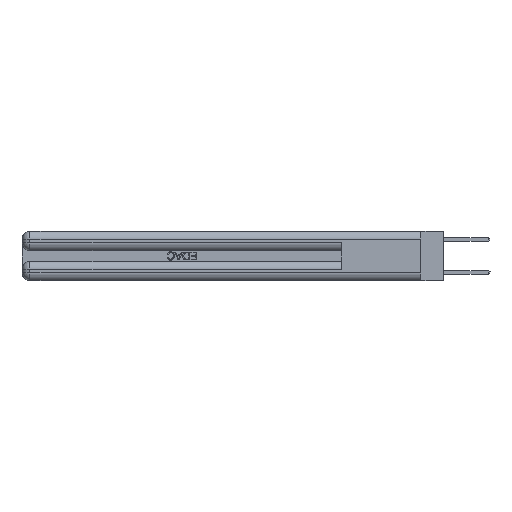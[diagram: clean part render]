
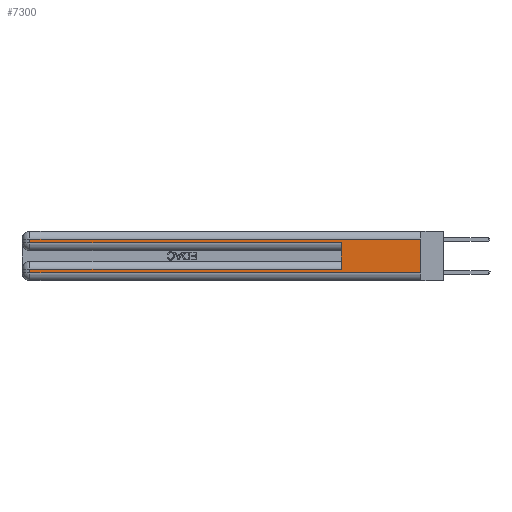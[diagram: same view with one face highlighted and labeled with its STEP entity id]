
A CAD part, left-side view. The second image highlights one B-rep face of the part: STEP entity #7300.
In plain terms, the highlighted planar face has unit normal (-1, 0, 0).
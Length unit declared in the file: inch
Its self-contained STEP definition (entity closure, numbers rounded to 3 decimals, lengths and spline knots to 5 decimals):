
#155 = CARTESIAN_POINT ( 'NONE',  ( 0., 2.94, 0.085 ) ) ;
#1651 = LINE ( 'NONE', #11303, #3616 ) ;
#1743 = CARTESIAN_POINT ( 'NONE',  ( 0., 0.6, 0.085 ) ) ;
#1828 = DIRECTION ( 'NONE',  ( 0., -1., 0. ) ) ;
#3302 = DIRECTION ( 'NONE',  ( 0., 0., -1. ) ) ;
#3616 = VECTOR ( 'NONE', #23784, 39.37008 ) ;
#3754 = EDGE_CURVE ( 'NONE', #8307, #14966, #9145, .T. ) ;
#5273 = LINE ( 'NONE', #17612, #16160 ) ;
#6534 = EDGE_CURVE ( 'NONE', #16472, #12339, #28603, .T. ) ;
#7300 = ADVANCED_FACE ( 'NONE', ( #20541 ), #13347, .F. ) ;
#7643 = CARTESIAN_POINT ( 'NONE',  ( 0., 2.94, 0.285 ) ) ;
#7908 = CARTESIAN_POINT ( 'NONE',  ( 0., 0., 0.31 ) ) ;
#8307 = VERTEX_POINT ( 'NONE', #27105 ) ;
#8525 = LINE ( 'NONE', #30599, #23856 ) ;
#8635 = EDGE_CURVE ( 'NONE', #29827, #12339, #8525, .T. ) ;
#9145 = LINE ( 'NONE', #21935, #31390 ) ;
#9627 = LINE ( 'NONE', #14282, #19614 ) ;
#10012 = ORIENTED_EDGE ( 'NONE', *, *, #6534, .T. ) ;
#10071 = CARTESIAN_POINT ( 'NONE',  ( 0., 2.94, 0.31 ) ) ;
#10777 = DIRECTION ( 'NONE',  ( 1., 0., 0. ) ) ;
#11303 = CARTESIAN_POINT ( 'NONE',  ( 0., 2.94, 0.37 ) ) ;
#12339 = VERTEX_POINT ( 'NONE', #18802 ) ;
#12485 = DIRECTION ( 'NONE',  ( 0., 1., 0. ) ) ;
#13347 = PLANE ( 'NONE',  #25347 ) ;
#13600 = VECTOR ( 'NONE', #3302, 39.37008 ) ;
#13696 = ORIENTED_EDGE ( 'NONE', *, *, #28185, .T. ) ;
#13989 = EDGE_CURVE ( 'NONE', #20534, #16472, #1651, .T. ) ;
#14158 = ORIENTED_EDGE ( 'NONE', *, *, #3754, .T. ) ;
#14263 = ORIENTED_EDGE ( 'NONE', *, *, #29992, .F. ) ;
#14282 = CARTESIAN_POINT ( 'NONE',  ( 0., 0., 0.37 ) ) ;
#14966 = VERTEX_POINT ( 'NONE', #19688 ) ;
#14976 = LINE ( 'NONE', #7908, #23549 ) ;
#16160 = VECTOR ( 'NONE', #12485, 39.37008 ) ;
#16472 = VERTEX_POINT ( 'NONE', #7643 ) ;
#17494 = EDGE_LOOP ( 'NONE', ( #14263, #13696, #19345, #10012, #31141, #26925, #22152, #14158 ) ) ;
#17612 = CARTESIAN_POINT ( 'NONE',  ( 0., 0., 0.085 ) ) ;
#18132 = DIRECTION ( 'NONE',  ( 0., 0., -1. ) ) ;
#18802 = CARTESIAN_POINT ( 'NONE',  ( 0., 0.6, 0.285 ) ) ;
#19345 = ORIENTED_EDGE ( 'NONE', *, *, #13989, .T. ) ;
#19614 = VECTOR ( 'NONE', #26897, 39.37008 ) ;
#19688 = CARTESIAN_POINT ( 'NONE',  ( 0., 0., 0.06 ) ) ;
#19989 = LINE ( 'NONE', #29738, #13600 ) ;
#20012 = EDGE_CURVE ( 'NONE', #29827, #24537, #5273, .T. ) ;
#20229 = CARTESIAN_POINT ( 'NONE',  ( 0., 0., 0.31 ) ) ;
#20429 = EDGE_CURVE ( 'NONE', #24537, #8307, #19989, .T. ) ;
#20534 = VERTEX_POINT ( 'NONE', #10071 ) ;
#20541 = FACE_OUTER_BOUND ( 'NONE', #17494, .T. ) ;
#20859 = DIRECTION ( 'NONE',  ( 0., 0., 1. ) ) ;
#21935 = CARTESIAN_POINT ( 'NONE',  ( 0., 0., 0.06 ) ) ;
#22152 = ORIENTED_EDGE ( 'NONE', *, *, #20429, .T. ) ;
#22859 = VECTOR ( 'NONE', #1828, 39.37008 ) ;
#23549 = VECTOR ( 'NONE', #29833, 39.37008 ) ;
#23784 = DIRECTION ( 'NONE',  ( 0., 0., -1. ) ) ;
#23856 = VECTOR ( 'NONE', #20859, 39.37008 ) ;
#24253 = CARTESIAN_POINT ( 'NONE',  ( 0., 0., 0.285 ) ) ;
#24537 = VERTEX_POINT ( 'NONE', #155 ) ;
#25347 = AXIS2_PLACEMENT_3D ( 'NONE', #28058, #10777, #18132 ) ;
#26897 = DIRECTION ( 'NONE',  ( 0., 0., -1. ) ) ;
#26925 = ORIENTED_EDGE ( 'NONE', *, *, #20012, .T. ) ;
#27105 = CARTESIAN_POINT ( 'NONE',  ( 0., 2.94, 0.06 ) ) ;
#28058 = CARTESIAN_POINT ( 'NONE',  ( 0., 0., 0.37 ) ) ;
#28185 = EDGE_CURVE ( 'NONE', #29767, #20534, #14976, .T. ) ;
#28603 = LINE ( 'NONE', #24253, #22859 ) ;
#29738 = CARTESIAN_POINT ( 'NONE',  ( 0., 2.94, 0.37 ) ) ;
#29767 = VERTEX_POINT ( 'NONE', #20229 ) ;
#29827 = VERTEX_POINT ( 'NONE', #1743 ) ;
#29833 = DIRECTION ( 'NONE',  ( 0., 1., 0. ) ) ;
#29992 = EDGE_CURVE ( 'NONE', #29767, #14966, #9627, .T. ) ;
#30599 = CARTESIAN_POINT ( 'NONE',  ( 0., 0.6, 0.145 ) ) ;
#31054 = DIRECTION ( 'NONE',  ( 0., -1., 0. ) ) ;
#31141 = ORIENTED_EDGE ( 'NONE', *, *, #8635, .F. ) ;
#31390 = VECTOR ( 'NONE', #31054, 39.37008 ) ;
